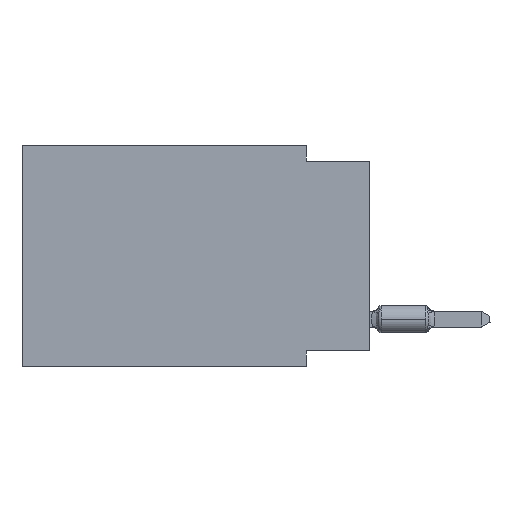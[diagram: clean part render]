
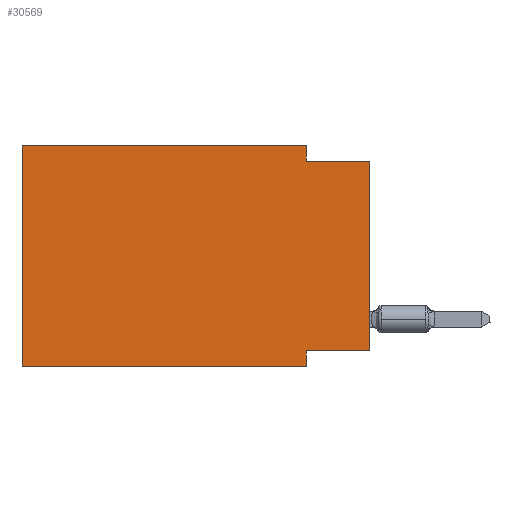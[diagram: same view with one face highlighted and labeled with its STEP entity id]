
A CAD part, left-side view. The second image highlights one B-rep face of the part: STEP entity #30569.
In plain terms, the highlighted planar face has unit normal (-1, 0, 0).
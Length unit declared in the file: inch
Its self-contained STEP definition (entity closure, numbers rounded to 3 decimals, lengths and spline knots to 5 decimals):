
#902 = CARTESIAN_POINT ( 'NONE',  ( 0., 0.1, -0.325 ) ) ;
#1743 = LINE ( 'NONE', #25455, #43242 ) ;
#2980 = CARTESIAN_POINT ( 'NONE',  ( 0., 0.55, 0. ) ) ;
#3902 = CARTESIAN_POINT ( 'NONE',  ( 0., 0.1, -0.35 ) ) ;
#5848 = CARTESIAN_POINT ( 'NONE',  ( 0., 0.1, -0.025 ) ) ;
#6308 = VERTEX_POINT ( 'NONE', #5848 ) ;
#8528 = ORIENTED_EDGE ( 'NONE', *, *, #74168, .T. ) ;
#9203 = LINE ( 'NONE', #69080, #68237 ) ;
#11462 = VECTOR ( 'NONE', #45750, 39.37008 ) ;
#11594 = EDGE_CURVE ( 'NONE', #31949, #52885, #76203, .T. ) ;
#12763 = ORIENTED_EDGE ( 'NONE', *, *, #59456, .F. ) ;
#14353 = VERTEX_POINT ( 'NONE', #38945 ) ;
#15479 = CARTESIAN_POINT ( 'NONE',  ( 0., 0., -0.025 ) ) ;
#15786 = DIRECTION ( 'NONE',  ( 0., 0., -1. ) ) ;
#17335 = CARTESIAN_POINT ( 'NONE',  ( 0., 0.55, 0. ) ) ;
#17742 = EDGE_CURVE ( 'NONE', #32774, #70221, #57403, .T. ) ;
#18881 = DIRECTION ( 'NONE',  ( 0., 0., -1. ) ) ;
#20566 = VERTEX_POINT ( 'NONE', #902 ) ;
#21736 = EDGE_CURVE ( 'NONE', #14353, #31949, #21965, .T. ) ;
#21965 = LINE ( 'NONE', #33612, #67649 ) ;
#22013 = CARTESIAN_POINT ( 'NONE',  ( 0., 0., 0. ) ) ;
#23163 = VECTOR ( 'NONE', #45049, 39.37008 ) ;
#24220 = EDGE_CURVE ( 'NONE', #6308, #70221, #56706, .T. ) ;
#25089 = LINE ( 'NONE', #76860, #75380 ) ;
#25455 = CARTESIAN_POINT ( 'NONE',  ( 0., 0., -0.325 ) ) ;
#26289 = ORIENTED_EDGE ( 'NONE', *, *, #11594, .F. ) ;
#26675 = DIRECTION ( 'NONE',  ( 1., 0., 0. ) ) ;
#27700 = AXIS2_PLACEMENT_3D ( 'NONE', #2980, #26675, #50418 ) ;
#30569 = ADVANCED_FACE ( 'NONE', ( #68688 ), #56250, .F. ) ;
#31949 = VERTEX_POINT ( 'NONE', #17335 ) ;
#32774 = VERTEX_POINT ( 'NONE', #70061 ) ;
#33612 = CARTESIAN_POINT ( 'NONE',  ( 0., 0.55, 0. ) ) ;
#34951 = DIRECTION ( 'NONE',  ( 0., -1., 0. ) ) ;
#35547 = DIRECTION ( 'NONE',  ( 0., -1., 0. ) ) ;
#36236 = ORIENTED_EDGE ( 'NONE', *, *, #21736, .F. ) ;
#36947 = ORIENTED_EDGE ( 'NONE', *, *, #24220, .F. ) ;
#38945 = CARTESIAN_POINT ( 'NONE',  ( 0., 0.55, -0.35 ) ) ;
#39728 = CARTESIAN_POINT ( 'NONE',  ( 0., 0., -0.025 ) ) ;
#40633 = DIRECTION ( 'NONE',  ( 0., 0., 1. ) ) ;
#43242 = VECTOR ( 'NONE', #72911, 39.37008 ) ;
#43648 = ORIENTED_EDGE ( 'NONE', *, *, #59138, .F. ) ;
#44253 = VERTEX_POINT ( 'NONE', #3902 ) ;
#45049 = DIRECTION ( 'NONE',  ( 0., -1., 0. ) ) ;
#45750 = DIRECTION ( 'NONE',  ( 0., 0., 1. ) ) ;
#48548 = EDGE_CURVE ( 'NONE', #52885, #6308, #25089, .T. ) ;
#50418 = DIRECTION ( 'NONE',  ( 0., 0., -1. ) ) ;
#52885 = VERTEX_POINT ( 'NONE', #57344 ) ;
#56250 = PLANE ( 'NONE',  #27700 ) ;
#56706 = LINE ( 'NONE', #15479, #23163 ) ;
#57239 = VECTOR ( 'NONE', #34951, 39.37008 ) ;
#57344 = CARTESIAN_POINT ( 'NONE',  ( 0., 0.1, 0. ) ) ;
#57403 = LINE ( 'NONE', #22013, #11462 ) ;
#58697 = ORIENTED_EDGE ( 'NONE', *, *, #48548, .F. ) ;
#59138 = EDGE_CURVE ( 'NONE', #20566, #44253, #9203, .T. ) ;
#59456 = EDGE_CURVE ( 'NONE', #32774, #20566, #1743, .T. ) ;
#67192 = VECTOR ( 'NONE', #35547, 39.37008 ) ;
#67649 = VECTOR ( 'NONE', #40633, 39.37008 ) ;
#68237 = VECTOR ( 'NONE', #15786, 39.37008 ) ;
#68688 = FACE_OUTER_BOUND ( 'NONE', #69864, .T. ) ;
#69059 = ORIENTED_EDGE ( 'NONE', *, *, #17742, .T. ) ;
#69080 = CARTESIAN_POINT ( 'NONE',  ( 0., 0.1, -0.35 ) ) ;
#69864 = EDGE_LOOP ( 'NONE', ( #69059, #36947, #58697, #26289, #36236, #8528, #43648, #12763 ) ) ;
#70061 = CARTESIAN_POINT ( 'NONE',  ( 0., 0., -0.325 ) ) ;
#70221 = VERTEX_POINT ( 'NONE', #39728 ) ;
#71339 = LINE ( 'NONE', #71722, #67192 ) ;
#71722 = CARTESIAN_POINT ( 'NONE',  ( 0., 0.55, -0.35 ) ) ;
#72911 = DIRECTION ( 'NONE',  ( 0., 1., 0. ) ) ;
#74168 = EDGE_CURVE ( 'NONE', #14353, #44253, #71339, .T. ) ;
#75055 = CARTESIAN_POINT ( 'NONE',  ( 0., 0.55, 0. ) ) ;
#75380 = VECTOR ( 'NONE', #18881, 39.37008 ) ;
#76203 = LINE ( 'NONE', #75055, #57239 ) ;
#76860 = CARTESIAN_POINT ( 'NONE',  ( 0., 0.1, 0. ) ) ;
